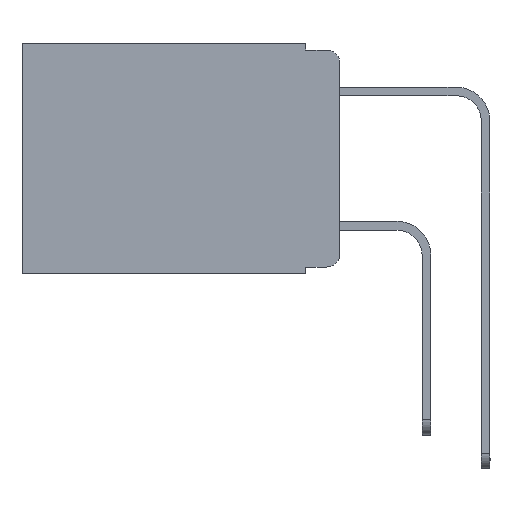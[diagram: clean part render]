
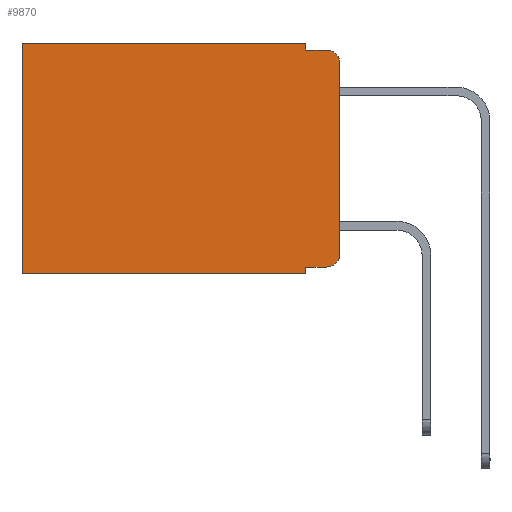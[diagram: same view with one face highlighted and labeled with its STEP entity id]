
A CAD part, left-side view. The second image highlights one B-rep face of the part: STEP entity #9870.
In plain terms, the highlighted planar face has unit normal (-1, 0, 0).
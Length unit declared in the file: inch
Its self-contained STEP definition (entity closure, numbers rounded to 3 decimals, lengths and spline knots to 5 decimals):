
#39 = VERTEX_POINT ( 'NONE', #4822 ) ;
#475 = DIRECTION ( 'NONE',  ( 1., 0., 0. ) ) ;
#603 = CARTESIAN_POINT ( 'NONE',  ( 0.298, 0., 0. ) ) ;
#616 = CIRCLE ( 'NONE', #2061, 0.02 ) ;
#870 = VECTOR ( 'NONE', #22240, 39.37008 ) ;
#1160 = DIRECTION ( 'NONE',  ( 0., 0., -1. ) ) ;
#1216 = VECTOR ( 'NONE', #19703, 39.37008 ) ;
#1343 = LINE ( 'NONE', #8242, #8104 ) ;
#1344 = EDGE_CURVE ( 'NONE', #6210, #7708, #616, .T. ) ;
#2061 = AXIS2_PLACEMENT_3D ( 'NONE', #3381, #5181, #3056 ) ;
#2522 = VECTOR ( 'NONE', #14866, 39.37008 ) ;
#2627 = LINE ( 'NONE', #4773, #2522 ) ;
#2670 = ORIENTED_EDGE ( 'NONE', *, *, #18235, .F. ) ;
#2972 = ORIENTED_EDGE ( 'NONE', *, *, #12836, .F. ) ;
#3056 = DIRECTION ( 'NONE',  ( 0., 0., -1. ) ) ;
#3133 = VERTEX_POINT ( 'NONE', #6751 ) ;
#3259 = VECTOR ( 'NONE', #18248, 39.37008 ) ;
#3327 = DIRECTION ( 'NONE',  ( 0., 0., -1. ) ) ;
#3381 = CARTESIAN_POINT ( 'NONE',  ( 0.298, 0.02, -0.313 ) ) ;
#3440 = VERTEX_POINT ( 'NONE', #7631 ) ;
#3452 = ORIENTED_EDGE ( 'NONE', *, *, #4012, .T. ) ;
#3804 = CARTESIAN_POINT ( 'NONE',  ( 0.298, 0.02, -0.333 ) ) ;
#4012 = EDGE_CURVE ( 'NONE', #3133, #6210, #9373, .T. ) ;
#4216 = PLANE ( 'NONE',  #11015 ) ;
#4371 = CARTESIAN_POINT ( 'NONE',  ( 0.298, 0., -0.313 ) ) ;
#4772 = ORIENTED_EDGE ( 'NONE', *, *, #20095, .F. ) ;
#4773 = CARTESIAN_POINT ( 'NONE',  ( 0.298, 0.051, 0. ) ) ;
#4822 = CARTESIAN_POINT ( 'NONE',  ( 0.298, 0.051, -0.343 ) ) ;
#5181 = DIRECTION ( 'NONE',  ( -1., 0., 0. ) ) ;
#5642 = CARTESIAN_POINT ( 'NONE',  ( 0.298, 0., 0. ) ) ;
#5836 = ORIENTED_EDGE ( 'NONE', *, *, #12975, .T. ) ;
#6069 = VERTEX_POINT ( 'NONE', #16988 ) ;
#6150 = DIRECTION ( 'NONE',  ( 0., -1., 0. ) ) ;
#6161 = CARTESIAN_POINT ( 'NONE',  ( 0.298, 0., -0.03 ) ) ;
#6210 = VERTEX_POINT ( 'NONE', #3804 ) ;
#6751 = CARTESIAN_POINT ( 'NONE',  ( 0.298, 0.051, -0.333 ) ) ;
#6791 = VECTOR ( 'NONE', #6150, 39.37008 ) ;
#6888 = ORIENTED_EDGE ( 'NONE', *, *, #16280, .F. ) ;
#6919 = EDGE_CURVE ( 'NONE', #15048, #16789, #21978, .T. ) ;
#7631 = CARTESIAN_POINT ( 'NONE',  ( 0.298, 0.051, 0. ) ) ;
#7708 = VERTEX_POINT ( 'NONE', #4371 ) ;
#7795 = AXIS2_PLACEMENT_3D ( 'NONE', #13398, #21949, #1160 ) ;
#8104 = VECTOR ( 'NONE', #16771, 39.37008 ) ;
#8168 = VECTOR ( 'NONE', #9349, 39.37008 ) ;
#8242 = CARTESIAN_POINT ( 'NONE',  ( 0.298, 0., 0. ) ) ;
#9158 = CARTESIAN_POINT ( 'NONE',  ( 0.298, 0.02, -0.01 ) ) ;
#9349 = DIRECTION ( 'NONE',  ( 0., 1., 0. ) ) ;
#9373 = LINE ( 'NONE', #19843, #3259 ) ;
#9870 = ADVANCED_FACE ( 'NONE', ( #19756 ), #4216, .F. ) ;
#10108 = CARTESIAN_POINT ( 'NONE',  ( 0.298, 0.051, 0. ) ) ;
#10165 = CARTESIAN_POINT ( 'NONE',  ( 0.298, 0.473, 0. ) ) ;
#10471 = CARTESIAN_POINT ( 'NONE',  ( 0.298, 0.051, -0.01 ) ) ;
#11015 = AXIS2_PLACEMENT_3D ( 'NONE', #603, #475, #21487 ) ;
#11067 = LINE ( 'NONE', #5642, #1216 ) ;
#11488 = CARTESIAN_POINT ( 'NONE',  ( 0.298, 0.473, -0.343 ) ) ;
#11834 = EDGE_LOOP ( 'NONE', ( #2972, #16796, #2670, #13419, #22069, #5836, #6888, #4772, #3452, #20247 ) ) ;
#11982 = EDGE_CURVE ( 'NONE', #3440, #6069, #11067, .T. ) ;
#12836 = EDGE_CURVE ( 'NONE', #15048, #7708, #1343, .T. ) ;
#12975 = EDGE_CURVE ( 'NONE', #6069, #14972, #20756, .T. ) ;
#13398 = CARTESIAN_POINT ( 'NONE',  ( 0.298, 0.02, -0.03 ) ) ;
#13419 = ORIENTED_EDGE ( 'NONE', *, *, #18383, .F. ) ;
#13560 = VERTEX_POINT ( 'NONE', #10471 ) ;
#14866 = DIRECTION ( 'NONE',  ( 0., 0., -1. ) ) ;
#14972 = VERTEX_POINT ( 'NONE', #11488 ) ;
#14992 = CARTESIAN_POINT ( 'NONE',  ( 0.298, 0.051, -0.01 ) ) ;
#15048 = VERTEX_POINT ( 'NONE', #6161 ) ;
#15667 = LINE ( 'NONE', #10108, #20976 ) ;
#16177 = LINE ( 'NONE', #18003, #8168 ) ;
#16280 = EDGE_CURVE ( 'NONE', #39, #14972, #16177, .T. ) ;
#16771 = DIRECTION ( 'NONE',  ( 0., 0., -1. ) ) ;
#16789 = VERTEX_POINT ( 'NONE', #9158 ) ;
#16796 = ORIENTED_EDGE ( 'NONE', *, *, #6919, .T. ) ;
#16988 = CARTESIAN_POINT ( 'NONE',  ( 0.298, 0.473, 0. ) ) ;
#18003 = CARTESIAN_POINT ( 'NONE',  ( 0.298, 0., -0.343 ) ) ;
#18182 = LINE ( 'NONE', #14992, #6791 ) ;
#18235 = EDGE_CURVE ( 'NONE', #13560, #16789, #18182, .T. ) ;
#18248 = DIRECTION ( 'NONE',  ( 0., -1., 0. ) ) ;
#18383 = EDGE_CURVE ( 'NONE', #3440, #13560, #15667, .T. ) ;
#19703 = DIRECTION ( 'NONE',  ( 0., 1., 0. ) ) ;
#19756 = FACE_OUTER_BOUND ( 'NONE', #11834, .T. ) ;
#19843 = CARTESIAN_POINT ( 'NONE',  ( 0.298, 0.051, -0.333 ) ) ;
#20095 = EDGE_CURVE ( 'NONE', #3133, #39, #2627, .T. ) ;
#20247 = ORIENTED_EDGE ( 'NONE', *, *, #1344, .T. ) ;
#20756 = LINE ( 'NONE', #10165, #870 ) ;
#20976 = VECTOR ( 'NONE', #3327, 39.37008 ) ;
#21487 = DIRECTION ( 'NONE',  ( 0., 0., -1. ) ) ;
#21949 = DIRECTION ( 'NONE',  ( -1., 0., 0. ) ) ;
#21978 = CIRCLE ( 'NONE', #7795, 0.02 ) ;
#22069 = ORIENTED_EDGE ( 'NONE', *, *, #11982, .T. ) ;
#22240 = DIRECTION ( 'NONE',  ( 0., 0., -1. ) ) ;
